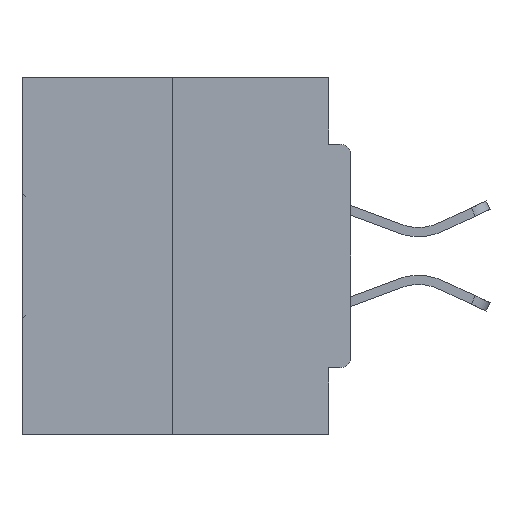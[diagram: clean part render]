
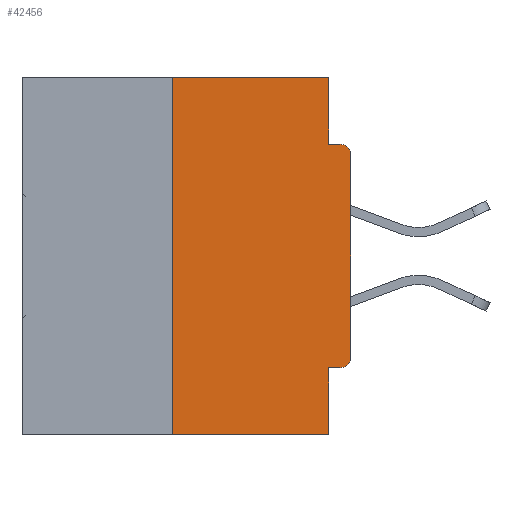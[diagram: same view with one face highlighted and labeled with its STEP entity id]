
A CAD part, left-side view. The second image highlights one B-rep face of the part: STEP entity #42456.
In plain terms, the highlighted planar face has unit normal (-1, 0, 0).
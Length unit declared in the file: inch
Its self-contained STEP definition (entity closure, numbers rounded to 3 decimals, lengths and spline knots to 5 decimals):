
#169 = ORIENTED_EDGE ( 'NONE', *, *, #37643, .T. ) ;
#1010 = VECTOR ( 'NONE', #38856, 39.37008 ) ;
#1901 = AXIS2_PLACEMENT_3D ( 'NONE', #12078, #32412, #32700 ) ;
#2948 = EDGE_CURVE ( 'NONE', #32476, #29543, #6117, .T. ) ;
#3955 = CARTESIAN_POINT ( 'NONE',  ( 0., 0.031, -0.5 ) ) ;
#4413 = VERTEX_POINT ( 'NONE', #38371 ) ;
#4996 = CARTESIAN_POINT ( 'NONE',  ( 0., 0.46, 0. ) ) ;
#6117 = LINE ( 'NONE', #24005, #27529 ) ;
#6493 = VECTOR ( 'NONE', #8559, 39.37008 ) ;
#6697 = LINE ( 'NONE', #4996, #40823 ) ;
#7741 = CARTESIAN_POINT ( 'NONE',  ( 0., 0.031, 0. ) ) ;
#8469 = DIRECTION ( 'NONE',  ( 0., -1., 0. ) ) ;
#8559 = DIRECTION ( 'NONE',  ( 0., -1., 0. ) ) ;
#8766 = LINE ( 'NONE', #3955, #17342 ) ;
#9094 = CARTESIAN_POINT ( 'NONE',  ( 0., 0.25, 0. ) ) ;
#9175 = CARTESIAN_POINT ( 'NONE',  ( 0., 0.25, 0. ) ) ;
#9355 = ORIENTED_EDGE ( 'NONE', *, *, #22943, .T. ) ;
#9596 = EDGE_CURVE ( 'NONE', #33926, #4413, #23987, .T. ) ;
#9642 = EDGE_CURVE ( 'NONE', #28102, #40814, #35770, .T. ) ;
#10031 = DIRECTION ( 'NONE',  ( 0., 0., -1. ) ) ;
#10817 = ORIENTED_EDGE ( 'NONE', *, *, #26004, .T. ) ;
#11765 = CARTESIAN_POINT ( 'NONE',  ( 0., 0.015, -0.0935 ) ) ;
#12001 = CARTESIAN_POINT ( 'NONE',  ( 0., 0.46, -0.5 ) ) ;
#12078 = CARTESIAN_POINT ( 'NONE',  ( 0., 0.46, 0. ) ) ;
#12124 = DIRECTION ( 'NONE',  ( 0., 0., 1. ) ) ;
#13082 = CARTESIAN_POINT ( 'NONE',  ( 0., 0.015, -0.3915 ) ) ;
#15708 = CARTESIAN_POINT ( 'NONE',  ( 0., 0.031, -0.5 ) ) ;
#15843 = ORIENTED_EDGE ( 'NONE', *, *, #36169, .F. ) ;
#16562 = DIRECTION ( 'NONE',  ( -1., 0., 0. ) ) ;
#16907 = ORIENTED_EDGE ( 'NONE', *, *, #43807, .F. ) ;
#17069 = ORIENTED_EDGE ( 'NONE', *, *, #9596, .T. ) ;
#17342 = VECTOR ( 'NONE', #31149, 39.37008 ) ;
#17476 = CARTESIAN_POINT ( 'NONE',  ( 0., 0.031, -0.4065 ) ) ;
#17639 = VECTOR ( 'NONE', #12124, 39.37008 ) ;
#18034 = VECTOR ( 'NONE', #18862, 39.37008 ) ;
#18597 = AXIS2_PLACEMENT_3D ( 'NONE', #13082, #16562, #40362 ) ;
#18655 = ORIENTED_EDGE ( 'NONE', *, *, #35875, .F. ) ;
#18862 = DIRECTION ( 'NONE',  ( 0., 0., 1. ) ) ;
#18900 = VECTOR ( 'NONE', #41987, 39.37008 ) ;
#20108 = LINE ( 'NONE', #9094, #18034 ) ;
#20358 = CIRCLE ( 'NONE', #18597, 0.015 ) ;
#20670 = DIRECTION ( 'NONE',  ( -1., 0., 0. ) ) ;
#22943 = EDGE_CURVE ( 'NONE', #4413, #29543, #38244, .T. ) ;
#23420 = CARTESIAN_POINT ( 'NONE',  ( 0., 0.031, -0.0935 ) ) ;
#23987 = LINE ( 'NONE', #29294, #17639 ) ;
#24005 = CARTESIAN_POINT ( 'NONE',  ( 0., 0., -0.0935 ) ) ;
#24149 = AXIS2_PLACEMENT_3D ( 'NONE', #37642, #20670, #10031 ) ;
#24836 = ORIENTED_EDGE ( 'NONE', *, *, #34870, .F. ) ;
#25994 = CARTESIAN_POINT ( 'NONE',  ( 0., 0., -0.3915 ) ) ;
#26004 = EDGE_CURVE ( 'NONE', #28102, #33926, #20358, .T. ) ;
#27529 = VECTOR ( 'NONE', #30560, 39.37008 ) ;
#28102 = VERTEX_POINT ( 'NONE', #39658 ) ;
#28951 = VERTEX_POINT ( 'NONE', #9175 ) ;
#29294 = CARTESIAN_POINT ( 'NONE',  ( 0., 0., 0. ) ) ;
#29543 = VERTEX_POINT ( 'NONE', #11765 ) ;
#29725 = ORIENTED_EDGE ( 'NONE', *, *, #9642, .F. ) ;
#30440 = VERTEX_POINT ( 'NONE', #41886 ) ;
#30474 = EDGE_LOOP ( 'NONE', ( #24836, #16907, #169, #18655, #29725, #10817, #17069, #9355, #34985, #15843 ) ) ;
#30560 = DIRECTION ( 'NONE',  ( 0., -1., 0. ) ) ;
#31149 = DIRECTION ( 'NONE',  ( 0., 0., -1. ) ) ;
#31884 = CARTESIAN_POINT ( 'NONE',  ( 0., 0.031, 0. ) ) ;
#32021 = CARTESIAN_POINT ( 'NONE',  ( 0., 0., -0.4065 ) ) ;
#32412 = DIRECTION ( 'NONE',  ( 1., 0., 0. ) ) ;
#32476 = VERTEX_POINT ( 'NONE', #23420 ) ;
#32700 = DIRECTION ( 'NONE',  ( 0., 0., -1. ) ) ;
#33926 = VERTEX_POINT ( 'NONE', #25994 ) ;
#34646 = VERTEX_POINT ( 'NONE', #7741 ) ;
#34870 = EDGE_CURVE ( 'NONE', #28951, #34646, #6697, .T. ) ;
#34985 = ORIENTED_EDGE ( 'NONE', *, *, #2948, .F. ) ;
#35694 = VERTEX_POINT ( 'NONE', #15708 ) ;
#35770 = LINE ( 'NONE', #32021, #1010 ) ;
#35875 = EDGE_CURVE ( 'NONE', #40814, #35694, #8766, .T. ) ;
#36169 = EDGE_CURVE ( 'NONE', #34646, #32476, #37016, .T. ) ;
#37016 = LINE ( 'NONE', #31884, #18900 ) ;
#37642 = CARTESIAN_POINT ( 'NONE',  ( 0., 0.015, -0.1085 ) ) ;
#37643 = EDGE_CURVE ( 'NONE', #30440, #35694, #41206, .T. ) ;
#38244 = CIRCLE ( 'NONE', #24149, 0.015 ) ;
#38371 = CARTESIAN_POINT ( 'NONE',  ( 0., 0., -0.1085 ) ) ;
#38856 = DIRECTION ( 'NONE',  ( 0., 1., 0. ) ) ;
#39658 = CARTESIAN_POINT ( 'NONE',  ( 0., 0.015, -0.4065 ) ) ;
#40362 = DIRECTION ( 'NONE',  ( 0., 0., -1. ) ) ;
#40426 = FACE_OUTER_BOUND ( 'NONE', #30474, .T. ) ;
#40814 = VERTEX_POINT ( 'NONE', #17476 ) ;
#40823 = VECTOR ( 'NONE', #8469, 39.37008 ) ;
#41206 = LINE ( 'NONE', #12001, #6493 ) ;
#41886 = CARTESIAN_POINT ( 'NONE',  ( 0., 0.25, -0.5 ) ) ;
#41987 = DIRECTION ( 'NONE',  ( 0., 0., -1. ) ) ;
#42456 = ADVANCED_FACE ( 'NONE', ( #40426 ), #42513, .F. ) ;
#42513 = PLANE ( 'NONE',  #1901 ) ;
#43807 = EDGE_CURVE ( 'NONE', #30440, #28951, #20108, .T. ) ;
